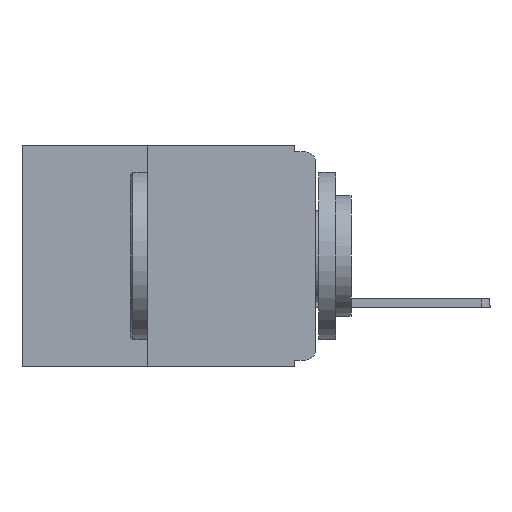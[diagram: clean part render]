
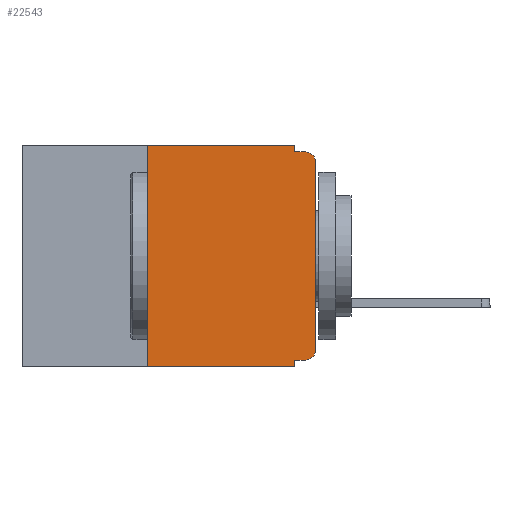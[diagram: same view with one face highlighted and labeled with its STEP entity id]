
A CAD part, left-side view. The second image highlights one B-rep face of the part: STEP entity #22543.
In plain terms, the highlighted planar face has unit normal (-1, 0, 0).
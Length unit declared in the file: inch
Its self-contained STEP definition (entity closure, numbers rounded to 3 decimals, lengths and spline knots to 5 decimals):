
#554 = VERTEX_POINT ( 'NONE', #23287 ) ;
#555 = VERTEX_POINT ( 'NONE', #13400 ) ;
#777 = DIRECTION ( 'NONE',  ( 1., 0., 0. ) ) ;
#2644 = VERTEX_POINT ( 'NONE', #24894 ) ;
#2654 = VECTOR ( 'NONE', #25504, 39.37008 ) ;
#2789 = EDGE_CURVE ( 'NONE', #13213, #555, #4791, .T. ) ;
#2826 = CARTESIAN_POINT ( 'NONE',  ( 0., 0.015, -0.025 ) ) ;
#2848 = EDGE_CURVE ( 'NONE', #3807, #2644, #14147, .T. ) ;
#3234 = ORIENTED_EDGE ( 'NONE', *, *, #2789, .F. ) ;
#3807 = VERTEX_POINT ( 'NONE', #21093 ) ;
#3963 = VERTEX_POINT ( 'NONE', #19164 ) ;
#4419 = AXIS2_PLACEMENT_3D ( 'NONE', #26712, #26658, #26625 ) ;
#4569 = VECTOR ( 'NONE', #22635, 39.37008 ) ;
#4580 = LINE ( 'NONE', #22318, #15916 ) ;
#4657 = CARTESIAN_POINT ( 'NONE',  ( 0., 0., -0.32 ) ) ;
#4791 = LINE ( 'NONE', #20058, #21112 ) ;
#4967 = DIRECTION ( 'NONE',  ( 0., 0., -1. ) ) ;
#5135 = PLANE ( 'NONE',  #12387 ) ;
#5230 = ORIENTED_EDGE ( 'NONE', *, *, #6267, .F. ) ;
#5273 = CARTESIAN_POINT ( 'NONE',  ( 0., 0.031, 0. ) ) ;
#5996 = EDGE_CURVE ( 'NONE', #24209, #3963, #6249, .T. ) ;
#6032 = ORIENTED_EDGE ( 'NONE', *, *, #19434, .T. ) ;
#6219 = ORIENTED_EDGE ( 'NONE', *, *, #10052, .T. ) ;
#6249 = CIRCLE ( 'NONE', #4419, 0.015 ) ;
#6267 = EDGE_CURVE ( 'NONE', #18517, #554, #4580, .T. ) ;
#6939 = AXIS2_PLACEMENT_3D ( 'NONE', #2826, #17748, #4967 ) ;
#7239 = DIRECTION ( 'NONE',  ( 0., 0., -1. ) ) ;
#7432 = CARTESIAN_POINT ( 'NONE',  ( 0., 0.25, -0.33 ) ) ;
#7684 = LINE ( 'NONE', #5273, #24044 ) ;
#7749 = VECTOR ( 'NONE', #18833, 39.37008 ) ;
#7811 = FACE_OUTER_BOUND ( 'NONE', #25737, .T. ) ;
#8959 = LINE ( 'NONE', #19110, #2654 ) ;
#9595 = DIRECTION ( 'NONE',  ( 0., 0., 1. ) ) ;
#9850 = ORIENTED_EDGE ( 'NONE', *, *, #15801, .T. ) ;
#10052 = EDGE_CURVE ( 'NONE', #17741, #554, #26065, .T. ) ;
#11093 = DIRECTION ( 'NONE',  ( 0., 1., 0. ) ) ;
#11526 = VECTOR ( 'NONE', #9595, 39.37008 ) ;
#12217 = LINE ( 'NONE', #7432, #11526 ) ;
#12358 = VERTEX_POINT ( 'NONE', #24851 ) ;
#12387 = AXIS2_PLACEMENT_3D ( 'NONE', #15770, #777, #7239 ) ;
#13213 = VERTEX_POINT ( 'NONE', #13221 ) ;
#13221 = CARTESIAN_POINT ( 'NONE',  ( 0., 0.25, 0. ) ) ;
#13400 = CARTESIAN_POINT ( 'NONE',  ( 0., 0.031, 0. ) ) ;
#13711 = ORIENTED_EDGE ( 'NONE', *, *, #23024, .F. ) ;
#14147 = LINE ( 'NONE', #18346, #7749 ) ;
#15459 = CARTESIAN_POINT ( 'NONE',  ( 0., 0.031, -0.01 ) ) ;
#15746 = ORIENTED_EDGE ( 'NONE', *, *, #2848, .F. ) ;
#15770 = CARTESIAN_POINT ( 'NONE',  ( 0., 0.437, 0. ) ) ;
#15801 = EDGE_CURVE ( 'NONE', #3963, #17741, #15902, .T. ) ;
#15902 = LINE ( 'NONE', #18362, #4569 ) ;
#15916 = VECTOR ( 'NONE', #22284, 39.37008 ) ;
#16277 = ORIENTED_EDGE ( 'NONE', *, *, #18667, .F. ) ;
#17163 = VECTOR ( 'NONE', #11093, 39.37008 ) ;
#17553 = CARTESIAN_POINT ( 'NONE',  ( 0., 0.015, -0.32 ) ) ;
#17741 = VERTEX_POINT ( 'NONE', #27545 ) ;
#17748 = DIRECTION ( 'NONE',  ( -1., 0., 0. ) ) ;
#18346 = CARTESIAN_POINT ( 'NONE',  ( 0., 0.031, -0.33 ) ) ;
#18362 = CARTESIAN_POINT ( 'NONE',  ( 0., 0., 0. ) ) ;
#18517 = VERTEX_POINT ( 'NONE', #15459 ) ;
#18667 = EDGE_CURVE ( 'NONE', #555, #18517, #7684, .T. ) ;
#18833 = DIRECTION ( 'NONE',  ( 0., 0., -1. ) ) ;
#19110 = CARTESIAN_POINT ( 'NONE',  ( 0., 0.437, -0.33 ) ) ;
#19164 = CARTESIAN_POINT ( 'NONE',  ( 0., 0., -0.305 ) ) ;
#19434 = EDGE_CURVE ( 'NONE', #12358, #2644, #8959, .T. ) ;
#19788 = DIRECTION ( 'NONE',  ( 0., -1., 0. ) ) ;
#20058 = CARTESIAN_POINT ( 'NONE',  ( 0., 0.437, 0. ) ) ;
#21093 = CARTESIAN_POINT ( 'NONE',  ( 0., 0.031, -0.32 ) ) ;
#21112 = VECTOR ( 'NONE', #19788, 39.37008 ) ;
#22284 = DIRECTION ( 'NONE',  ( 0., -1., 0. ) ) ;
#22318 = CARTESIAN_POINT ( 'NONE',  ( 0., 0., -0.01 ) ) ;
#22322 = DIRECTION ( 'NONE',  ( 0., 0., -1. ) ) ;
#22543 = ADVANCED_FACE ( 'NONE', ( #7811 ), #5135, .F. ) ;
#22606 = EDGE_CURVE ( 'NONE', #12358, #13213, #12217, .T. ) ;
#22635 = DIRECTION ( 'NONE',  ( 0., 0., 1. ) ) ;
#22824 = LINE ( 'NONE', #4657, #17163 ) ;
#23024 = EDGE_CURVE ( 'NONE', #24209, #3807, #22824, .T. ) ;
#23287 = CARTESIAN_POINT ( 'NONE',  ( 0., 0.015, -0.01 ) ) ;
#23869 = ORIENTED_EDGE ( 'NONE', *, *, #5996, .T. ) ;
#24044 = VECTOR ( 'NONE', #22322, 39.37008 ) ;
#24209 = VERTEX_POINT ( 'NONE', #17553 ) ;
#24251 = ORIENTED_EDGE ( 'NONE', *, *, #22606, .F. ) ;
#24851 = CARTESIAN_POINT ( 'NONE',  ( 0., 0.25, -0.33 ) ) ;
#24894 = CARTESIAN_POINT ( 'NONE',  ( 0., 0.031, -0.33 ) ) ;
#25504 = DIRECTION ( 'NONE',  ( 0., -1., 0. ) ) ;
#25737 = EDGE_LOOP ( 'NONE', ( #9850, #6219, #5230, #16277, #3234, #24251, #6032, #15746, #13711, #23869 ) ) ;
#26065 = CIRCLE ( 'NONE', #6939, 0.015 ) ;
#26625 = DIRECTION ( 'NONE',  ( 0., 0., -1. ) ) ;
#26658 = DIRECTION ( 'NONE',  ( -1., 0., 0. ) ) ;
#26712 = CARTESIAN_POINT ( 'NONE',  ( 0., 0.015, -0.305 ) ) ;
#27545 = CARTESIAN_POINT ( 'NONE',  ( 0., 0., -0.025 ) ) ;
